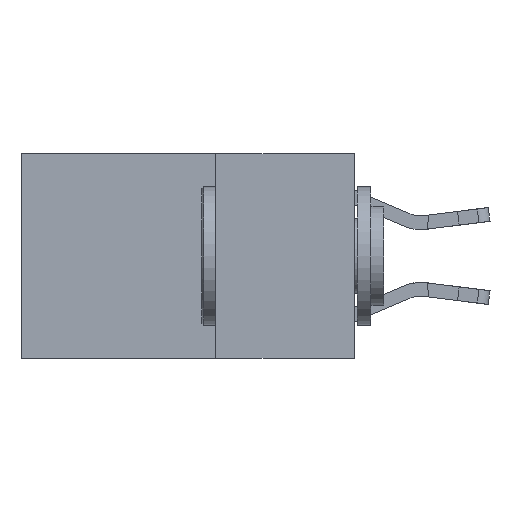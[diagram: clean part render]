
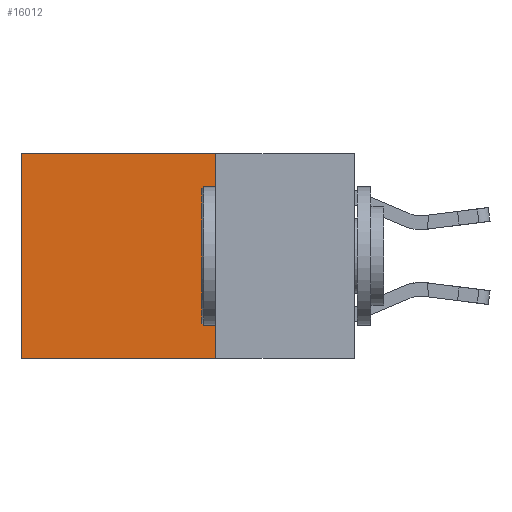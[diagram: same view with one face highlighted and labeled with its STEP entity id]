
A CAD part, left-side view. The second image highlights one B-rep face of the part: STEP entity #16012.
In plain terms, the highlighted planar face has unit normal (-1, 0, 0).
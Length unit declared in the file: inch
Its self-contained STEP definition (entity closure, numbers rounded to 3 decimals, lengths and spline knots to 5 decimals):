
#954 = FACE_OUTER_BOUND ( 'NONE', #9779, .T. ) ;
#1206 = EDGE_CURVE ( 'NONE', #4772, #11600, #4584, .T. ) ;
#1379 = VECTOR ( 'NONE', #17943, 39.37008 ) ;
#2999 = DIRECTION ( 'NONE',  ( 1., 0., 0. ) ) ;
#4584 = LINE ( 'NONE', #18274, #5095 ) ;
#4772 = VERTEX_POINT ( 'NONE', #21959 ) ;
#4865 = ORIENTED_EDGE ( 'NONE', *, *, #5576, .T. ) ;
#5095 = VECTOR ( 'NONE', #18514, 39.37008 ) ;
#5321 = LINE ( 'NONE', #12987, #7500 ) ;
#5576 = EDGE_CURVE ( 'NONE', #11600, #15650, #5321, .T. ) ;
#6548 = CARTESIAN_POINT ( 'NONE',  ( 0.2625, 0.25, -0.37 ) ) ;
#7500 = VECTOR ( 'NONE', #22692, 39.37008 ) ;
#9779 = EDGE_LOOP ( 'NONE', ( #4865, #22115, #13570, #21189 ) ) ;
#10416 = DIRECTION ( 'NONE',  ( 0., 1., 0. ) ) ;
#10519 = EDGE_CURVE ( 'NONE', #18922, #15650, #20101, .T. ) ;
#10925 = DIRECTION ( 'NONE',  ( 0., 0., -1. ) ) ;
#11029 = VECTOR ( 'NONE', #10416, 39.37008 ) ;
#11600 = VERTEX_POINT ( 'NONE', #22807 ) ;
#12987 = CARTESIAN_POINT ( 'NONE',  ( 0.2625, 0.6, 0. ) ) ;
#13501 = CARTESIAN_POINT ( 'NONE',  ( 0.2625, 0.6, -0.37 ) ) ;
#13570 = ORIENTED_EDGE ( 'NONE', *, *, #16231, .F. ) ;
#15650 = VERTEX_POINT ( 'NONE', #13501 ) ;
#16012 = ADVANCED_FACE ( 'NONE', ( #954 ), #16549, .F. ) ;
#16231 = EDGE_CURVE ( 'NONE', #4772, #18922, #23935, .T. ) ;
#16549 = PLANE ( 'NONE',  #18919 ) ;
#17943 = DIRECTION ( 'NONE',  ( 0., 0., -1. ) ) ;
#18274 = CARTESIAN_POINT ( 'NONE',  ( 0.2625, 0.25, 0. ) ) ;
#18514 = DIRECTION ( 'NONE',  ( 0., 1., 0. ) ) ;
#18919 = AXIS2_PLACEMENT_3D ( 'NONE', #24334, #2999, #10925 ) ;
#18922 = VERTEX_POINT ( 'NONE', #6548 ) ;
#20073 = CARTESIAN_POINT ( 'NONE',  ( 0.2625, 0.25, 0. ) ) ;
#20101 = LINE ( 'NONE', #23712, #11029 ) ;
#21189 = ORIENTED_EDGE ( 'NONE', *, *, #1206, .T. ) ;
#21959 = CARTESIAN_POINT ( 'NONE',  ( 0.2625, 0.25, 0. ) ) ;
#22115 = ORIENTED_EDGE ( 'NONE', *, *, #10519, .F. ) ;
#22692 = DIRECTION ( 'NONE',  ( 0., 0., -1. ) ) ;
#22807 = CARTESIAN_POINT ( 'NONE',  ( 0.2625, 0.6, 0. ) ) ;
#23712 = CARTESIAN_POINT ( 'NONE',  ( 0.2625, 0.25, -0.37 ) ) ;
#23935 = LINE ( 'NONE', #20073, #1379 ) ;
#24334 = CARTESIAN_POINT ( 'NONE',  ( 0.2625, 0.25, 0. ) ) ;
